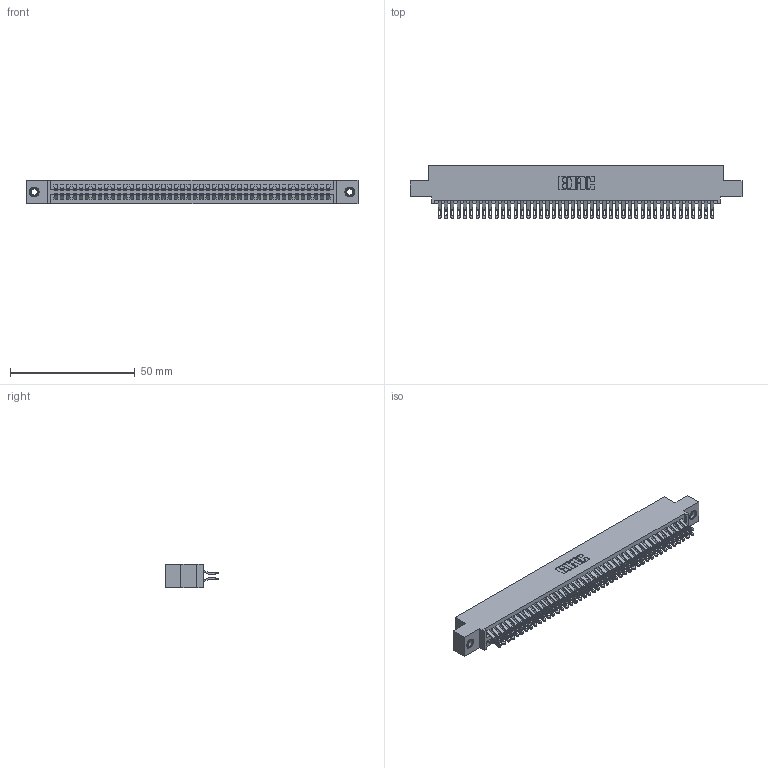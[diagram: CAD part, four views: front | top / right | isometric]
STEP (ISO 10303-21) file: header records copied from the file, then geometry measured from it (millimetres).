
FILE_DESCRIPTION (( 'STEP AP203' ), '1' );
FILE_NAME ('395-088-555-507.STEP', '2018-11-29T00:58:50', ( '' ), ( '' ), 'SwSTEP 2.0', 'SolidWorks 2016', '' );
FILE_SCHEMA (( 'CONFIG_CONTROL_DESIGN' ));
Length unit declared in the file: inch
Products named in the file (4): 395-088-555-507; 345 Part_0.110 Offset - 0.156 Dia-TI; 345-292-001_555 Tail; 345-250-001_345-250-005-103
Assembly tree (91 placements, depth 2):
  395-088-555-507
    345 Part_0.110 Offset - 0.156 Dia-TI
    345-292-001_555 Tail  x88
    345-250-001_345-250-005-103  x2
Bounding box: 132.97 x 21.13 x 9.4 mm (x, y, z)
Volume: 13103.7 mm3; surface area: 20416.7 mm2
Topology: 91 solids, 91 shells, 5118 faces, 16065 edges, 10702 vertices
Faces by surface type: plane 2844, cylinder 2258, cone 12, torus 4
Entity records: 35898 total; most frequent: CARTESIAN_POINT 6033, ORIENTED_EDGE 5930, DIRECTION 5311, EDGE_CURVE 2965, LINE 2617, VECTOR 2617, VERTEX_POINT 1972, AXIS2_PLACEMENT_3D 1347
